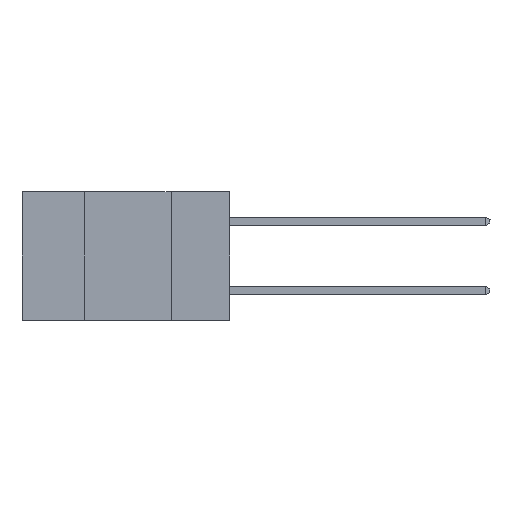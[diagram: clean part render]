
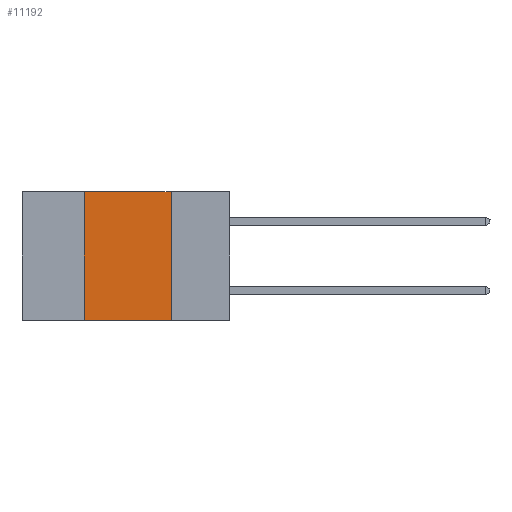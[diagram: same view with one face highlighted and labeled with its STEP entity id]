
A CAD part, left-side view. The second image highlights one B-rep face of the part: STEP entity #11192.
In plain terms, the highlighted planar face has unit normal (-1, 0, 0).
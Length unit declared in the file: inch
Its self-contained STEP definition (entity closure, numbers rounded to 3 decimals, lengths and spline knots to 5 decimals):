
#287 = CARTESIAN_POINT ( 'NONE',  ( 0., 0.6, 0. ) ) ;
#1425 = LINE ( 'NONE', #287, #11511 ) ;
#1609 = AXIS2_PLACEMENT_3D ( 'NONE', #9292, #13600, #3908 ) ;
#1740 = VERTEX_POINT ( 'NONE', #4577 ) ;
#1852 = CARTESIAN_POINT ( 'NONE',  ( 0., 0.42, -0.37 ) ) ;
#1890 = VERTEX_POINT ( 'NONE', #12442 ) ;
#1972 = EDGE_LOOP ( 'NONE', ( #10731, #10642, #8190, #6562 ) ) ;
#2754 = VECTOR ( 'NONE', #13902, 39.37008 ) ;
#3908 = DIRECTION ( 'NONE',  ( 0., 0., -1. ) ) ;
#4468 = VERTEX_POINT ( 'NONE', #12388 ) ;
#4577 = CARTESIAN_POINT ( 'NONE',  ( 0., 0.42, 0. ) ) ;
#5274 = LINE ( 'NONE', #7134, #2754 ) ;
#5826 = EDGE_CURVE ( 'NONE', #1740, #4468, #1425, .T. ) ;
#6084 = EDGE_CURVE ( 'NONE', #7224, #1740, #12742, .T. ) ;
#6192 = EDGE_CURVE ( 'NONE', #4468, #1890, #13016, .T. ) ;
#6562 = ORIENTED_EDGE ( 'NONE', *, *, #8968, .T. ) ;
#7090 = PLANE ( 'NONE',  #1609 ) ;
#7134 = CARTESIAN_POINT ( 'NONE',  ( 0., 0.6, -0.37 ) ) ;
#7224 = VERTEX_POINT ( 'NONE', #1852 ) ;
#7288 = CARTESIAN_POINT ( 'NONE',  ( 0., 0.17, -0.37 ) ) ;
#8009 = DIRECTION ( 'NONE',  ( 0., -1., 0. ) ) ;
#8151 = FACE_OUTER_BOUND ( 'NONE', #1972, .T. ) ;
#8190 = ORIENTED_EDGE ( 'NONE', *, *, #6084, .F. ) ;
#8968 = EDGE_CURVE ( 'NONE', #7224, #1890, #5274, .T. ) ;
#9292 = CARTESIAN_POINT ( 'NONE',  ( 0., 0.6, 0. ) ) ;
#10555 = DIRECTION ( 'NONE',  ( 0., 0., 1. ) ) ;
#10642 = ORIENTED_EDGE ( 'NONE', *, *, #5826, .F. ) ;
#10731 = ORIENTED_EDGE ( 'NONE', *, *, #6192, .F. ) ;
#11192 = ADVANCED_FACE ( 'NONE', ( #8151 ), #7090, .F. ) ;
#11511 = VECTOR ( 'NONE', #8009, 39.37008 ) ;
#11624 = DIRECTION ( 'NONE',  ( 0., 0., -1. ) ) ;
#11829 = CARTESIAN_POINT ( 'NONE',  ( 0., 0.42, -0.37 ) ) ;
#12388 = CARTESIAN_POINT ( 'NONE',  ( 0., 0.17, 0. ) ) ;
#12407 = VECTOR ( 'NONE', #10555, 39.37008 ) ;
#12442 = CARTESIAN_POINT ( 'NONE',  ( 0., 0.17, -0.37 ) ) ;
#12742 = LINE ( 'NONE', #11829, #12407 ) ;
#13016 = LINE ( 'NONE', #7288, #13748 ) ;
#13600 = DIRECTION ( 'NONE',  ( 1., 0., 0. ) ) ;
#13748 = VECTOR ( 'NONE', #11624, 39.37008 ) ;
#13902 = DIRECTION ( 'NONE',  ( 0., -1., 0. ) ) ;
